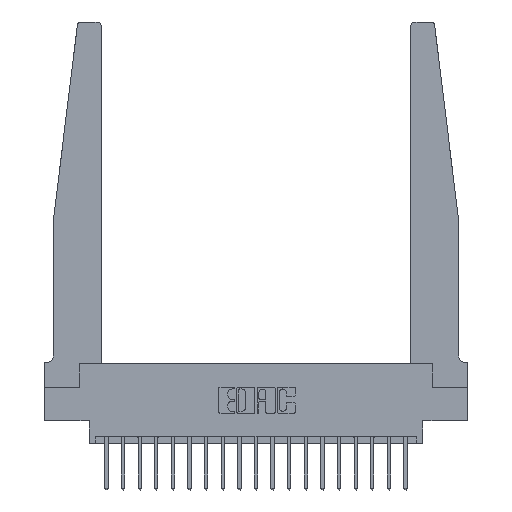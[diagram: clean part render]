
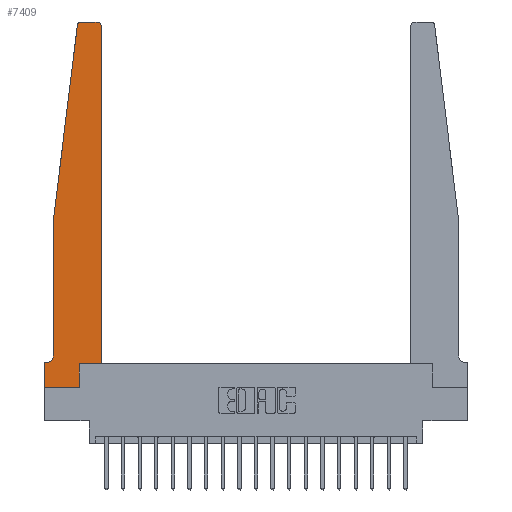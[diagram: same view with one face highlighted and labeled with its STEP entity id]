
A CAD part, top view. The second image highlights one B-rep face of the part: STEP entity #7409.
In plain terms, the highlighted planar face has unit normal (0, 0, 1).
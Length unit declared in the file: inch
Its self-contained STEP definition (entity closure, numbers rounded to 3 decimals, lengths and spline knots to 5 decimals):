
#1 = AXIS2_PLACEMENT_3D ( 'NONE', #10270, #6694, #5110 ) ;
#58 = EDGE_CURVE ( 'NONE', #17189, #12421, #16732, .T. ) ;
#182 = VECTOR ( 'NONE', #1505, 39.37008 ) ;
#863 = ORIENTED_EDGE ( 'NONE', *, *, #7830, .T. ) ;
#946 = VERTEX_POINT ( 'NONE', #10850 ) ;
#1048 = CARTESIAN_POINT ( 'NONE',  ( 0.065, 1.25, 0.37 ) ) ;
#1138 = DIRECTION ( 'NONE',  ( 0., 1., 0. ) ) ;
#1254 = VECTOR ( 'NONE', #3819, 39.37008 ) ;
#1505 = DIRECTION ( 'NONE',  ( 1., 0., 0. ) ) ;
#1687 = DIRECTION ( 'NONE',  ( 0., 0., 1. ) ) ;
#2147 = CARTESIAN_POINT ( 'NONE',  ( 0.065, 0.1875, 0.37 ) ) ;
#2249 = AXIS2_PLACEMENT_3D ( 'NONE', #16180, #3513, #16494 ) ;
#2341 = CIRCLE ( 'NONE', #1, 0.05 ) ;
#2514 = LINE ( 'NONE', #2731, #6551 ) ;
#2516 = LINE ( 'NONE', #7463, #17774 ) ;
#2731 = CARTESIAN_POINT ( 'NONE',  ( 0.425, 0.18, 0.37 ) ) ;
#3090 = LINE ( 'NONE', #11317, #12336 ) ;
#3513 = DIRECTION ( 'NONE',  ( 0., 0., 1. ) ) ;
#3795 = EDGE_CURVE ( 'NONE', #11036, #946, #3090, .T. ) ;
#3819 = DIRECTION ( 'NONE',  ( 0., -1., 0. ) ) ;
#3836 = DIRECTION ( 'NONE',  ( -1., 0., 0. ) ) ;
#3885 = DIRECTION ( 'NONE',  ( -0.122, -0.992, 0. ) ) ;
#4513 = EDGE_CURVE ( 'NONE', #14940, #8913, #7044, .T. ) ;
#4603 = EDGE_CURVE ( 'NONE', #8913, #19213, #2516, .T. ) ;
#4613 = LINE ( 'NONE', #14226, #13612 ) ;
#4721 = CARTESIAN_POINT ( 'NONE',  ( 0.425, 0.18, 0.37 ) ) ;
#5110 = DIRECTION ( 'NONE',  ( -1., 0., 0. ) ) ;
#5263 = CARTESIAN_POINT ( 'NONE',  ( 0.24675, 2.72367, 0.37 ) ) ;
#5333 = EDGE_CURVE ( 'NONE', #11514, #9370, #16928, .T. ) ;
#5403 = CARTESIAN_POINT ( 'NONE',  ( 0., 0., 0.37 ) ) ;
#6311 = VECTOR ( 'NONE', #3885, 39.37008 ) ;
#6366 = VERTEX_POINT ( 'NONE', #15256 ) ;
#6551 = VECTOR ( 'NONE', #12236, 39.37008 ) ;
#6694 = DIRECTION ( 'NONE',  ( 0., 0., -1. ) ) ;
#6808 = AXIS2_PLACEMENT_3D ( 'NONE', #8510, #1687, #13092 ) ;
#6892 = VECTOR ( 'NONE', #18549, 39.37008 ) ;
#7044 = LINE ( 'NONE', #1048, #6311 ) ;
#7252 = CARTESIAN_POINT ( 'NONE',  ( 0., 0.1875, 0.37 ) ) ;
#7409 = ADVANCED_FACE ( 'NONE', ( #16250 ), #16559, .T. ) ;
#7463 = CARTESIAN_POINT ( 'NONE',  ( 0.065, 1.25, 0.37 ) ) ;
#7830 = EDGE_CURVE ( 'NONE', #19213, #11514, #2341, .T. ) ;
#7891 = ORIENTED_EDGE ( 'NONE', *, *, #15212, .T. ) ;
#7931 = DIRECTION ( 'NONE',  ( 0., 1., 0. ) ) ;
#8255 = ORIENTED_EDGE ( 'NONE', *, *, #5333, .T. ) ;
#8510 = CARTESIAN_POINT ( 'NONE',  ( 0., 0.1875, 0.37 ) ) ;
#8897 = VERTEX_POINT ( 'NONE', #4721 ) ;
#8913 = VERTEX_POINT ( 'NONE', #16013 ) ;
#9321 = ORIENTED_EDGE ( 'NONE', *, *, #14164, .T. ) ;
#9370 = VERTEX_POINT ( 'NONE', #7252 ) ;
#9445 = CARTESIAN_POINT ( 'NONE',  ( 0.27653, 2.75, 0.37 ) ) ;
#9448 = EDGE_LOOP ( 'NONE', ( #7891, #16569, #17313, #20643, #863, #8255, #18927, #20234, #14401, #12143, #9321, #9628 ) ) ;
#9628 = ORIENTED_EDGE ( 'NONE', *, *, #58, .T. ) ;
#10112 = EDGE_CURVE ( 'NONE', #6366, #11036, #15868, .T. ) ;
#10187 = EDGE_CURVE ( 'NONE', #11376, #14940, #11720, .T. ) ;
#10270 = CARTESIAN_POINT ( 'NONE',  ( 0.015, 0.2375, 0.37 ) ) ;
#10850 = CARTESIAN_POINT ( 'NONE',  ( 0.2605, 0.18, 0.37 ) ) ;
#11036 = VERTEX_POINT ( 'NONE', #18317 ) ;
#11178 = CARTESIAN_POINT ( 'NONE',  ( 0.065, 0.2375, 0.37 ) ) ;
#11317 = CARTESIAN_POINT ( 'NONE',  ( 0.2605, 0.18, 0.37 ) ) ;
#11376 = VERTEX_POINT ( 'NONE', #9445 ) ;
#11514 = VERTEX_POINT ( 'NONE', #13458 ) ;
#11650 = LINE ( 'NONE', #5403, #1254 ) ;
#11720 = CIRCLE ( 'NONE', #2249, 0.03 ) ;
#12143 = ORIENTED_EDGE ( 'NONE', *, *, #15210, .T. ) ;
#12236 = DIRECTION ( 'NONE',  ( 1., 0., 0. ) ) ;
#12336 = VECTOR ( 'NONE', #7931, 39.37008 ) ;
#12421 = VERTEX_POINT ( 'NONE', #14109 ) ;
#13092 = DIRECTION ( 'NONE',  ( 1., 0., 0. ) ) ;
#13458 = CARTESIAN_POINT ( 'NONE',  ( 0.015, 0.1875, 0.37 ) ) ;
#13547 = DIRECTION ( 'NONE',  ( 0., 0., 1. ) ) ;
#13612 = VECTOR ( 'NONE', #1138, 39.37008 ) ;
#14109 = CARTESIAN_POINT ( 'NONE',  ( 0.395, 2.75, 0.37 ) ) ;
#14164 = EDGE_CURVE ( 'NONE', #8897, #17189, #4613, .T. ) ;
#14226 = CARTESIAN_POINT ( 'NONE',  ( 0.425, 0.18, 0.37 ) ) ;
#14401 = ORIENTED_EDGE ( 'NONE', *, *, #3795, .T. ) ;
#14940 = VERTEX_POINT ( 'NONE', #5263 ) ;
#15124 = VECTOR ( 'NONE', #3836, 39.37008 ) ;
#15210 = EDGE_CURVE ( 'NONE', #946, #8897, #2514, .T. ) ;
#15212 = EDGE_CURVE ( 'NONE', #12421, #11376, #15506, .T. ) ;
#15256 = CARTESIAN_POINT ( 'NONE',  ( 0., 0., 0.37 ) ) ;
#15506 = LINE ( 'NONE', #18658, #6892 ) ;
#15868 = LINE ( 'NONE', #15964, #182 ) ;
#15964 = CARTESIAN_POINT ( 'NONE',  ( 0., 0., 0.37 ) ) ;
#16013 = CARTESIAN_POINT ( 'NONE',  ( 0.065, 1.25, 0.37 ) ) ;
#16180 = CARTESIAN_POINT ( 'NONE',  ( 0.27653, 2.72, 0.37 ) ) ;
#16250 = FACE_OUTER_BOUND ( 'NONE', #9448, .T. ) ;
#16494 = DIRECTION ( 'NONE',  ( 1., 0., 0. ) ) ;
#16559 = PLANE ( 'NONE',  #6808 ) ;
#16569 = ORIENTED_EDGE ( 'NONE', *, *, #10187, .T. ) ;
#16732 = CIRCLE ( 'NONE', #19430, 0.03 ) ;
#16928 = LINE ( 'NONE', #2147, #15124 ) ;
#16975 = DIRECTION ( 'NONE',  ( 0., -1., 0. ) ) ;
#17189 = VERTEX_POINT ( 'NONE', #20846 ) ;
#17313 = ORIENTED_EDGE ( 'NONE', *, *, #4513, .T. ) ;
#17774 = VECTOR ( 'NONE', #16975, 39.37008 ) ;
#18317 = CARTESIAN_POINT ( 'NONE',  ( 0.2605, 0., 0.37 ) ) ;
#18549 = DIRECTION ( 'NONE',  ( -1., 0., 0. ) ) ;
#18658 = CARTESIAN_POINT ( 'NONE',  ( 0.25, 2.75, 0.37 ) ) ;
#18927 = ORIENTED_EDGE ( 'NONE', *, *, #20117, .T. ) ;
#19213 = VERTEX_POINT ( 'NONE', #11178 ) ;
#19430 = AXIS2_PLACEMENT_3D ( 'NONE', #19773, #13547, #20191 ) ;
#19773 = CARTESIAN_POINT ( 'NONE',  ( 0.395, 2.72, 0.37 ) ) ;
#20117 = EDGE_CURVE ( 'NONE', #9370, #6366, #11650, .T. ) ;
#20191 = DIRECTION ( 'NONE',  ( 1., 0., 0. ) ) ;
#20234 = ORIENTED_EDGE ( 'NONE', *, *, #10112, .T. ) ;
#20643 = ORIENTED_EDGE ( 'NONE', *, *, #4603, .T. ) ;
#20846 = CARTESIAN_POINT ( 'NONE',  ( 0.425, 2.72, 0.37 ) ) ;
